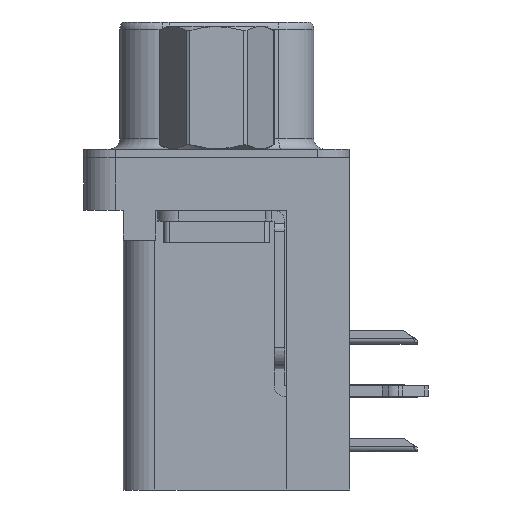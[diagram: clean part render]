
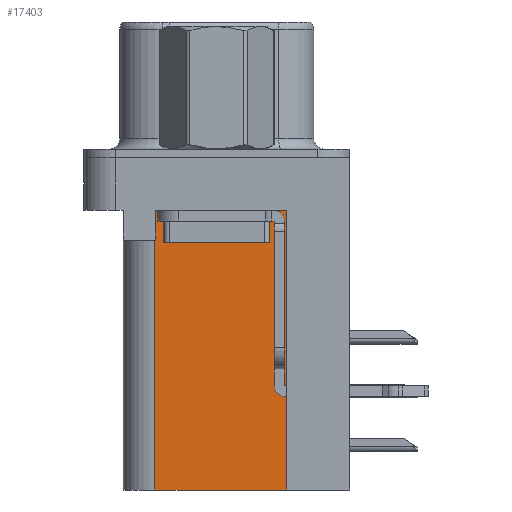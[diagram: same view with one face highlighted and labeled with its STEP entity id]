
A CAD part, left-side view. The second image highlights one B-rep face of the part: STEP entity #17403.
In plain terms, the highlighted planar face has unit normal (-1, 0, 0).
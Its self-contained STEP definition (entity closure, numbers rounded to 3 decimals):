
#1299 = ORIENTED_EDGE ( 'NONE', *, *, #2107, .T. ) ;
#1419 = ORIENTED_EDGE ( 'NONE', *, *, #11185, .T. ) ;
#1786 = LINE ( 'NONE', #12034, #20273 ) ;
#1880 = VECTOR ( 'NONE', #23965, 1000. ) ;
#2056 = EDGE_CURVE ( 'NONE', #6835, #28016, #26701, .T. ) ;
#2107 = EDGE_CURVE ( 'NONE', #3809, #8611, #20154, .T. ) ;
#2219 = CARTESIAN_POINT ( 'NONE',  ( 3.765, 2.925, -15.7 ) ) ;
#3132 = DIRECTION ( 'NONE',  ( 0., 0., -1. ) ) ;
#3398 = ORIENTED_EDGE ( 'NONE', *, *, #2056, .F. ) ;
#3809 = VERTEX_POINT ( 'NONE', #26616 ) ;
#4147 = CARTESIAN_POINT ( 'NONE',  ( 3.765, 2.925, -3.9 ) ) ;
#5010 = CARTESIAN_POINT ( 'NONE',  ( 3.765, 2.925, -15.7 ) ) ;
#6704 = LINE ( 'NONE', #8851, #17920 ) ;
#6835 = VERTEX_POINT ( 'NONE', #2219 ) ;
#7453 = CARTESIAN_POINT ( 'NONE',  ( 3.765, -3.295, -15.7 ) ) ;
#7613 = EDGE_CURVE ( 'NONE', #17355, #6835, #1786, .T. ) ;
#8280 = VECTOR ( 'NONE', #3132, 1000. ) ;
#8340 = CARTESIAN_POINT ( 'NONE',  ( 3.765, 2.895, -3.9 ) ) ;
#8611 = VERTEX_POINT ( 'NONE', #8340 ) ;
#8851 = CARTESIAN_POINT ( 'NONE',  ( 3.765, 0., -3.9 ) ) ;
#9215 = CARTESIAN_POINT ( 'NONE',  ( 3.765, -3.295, -2.5 ) ) ;
#10832 = EDGE_CURVE ( 'NONE', #17355, #16299, #27985, .T. ) ;
#11127 = DIRECTION ( 'NONE',  ( 0., 1., 0. ) ) ;
#11185 = EDGE_CURVE ( 'NONE', #16299, #3809, #20374, .T. ) ;
#12034 = CARTESIAN_POINT ( 'NONE',  ( 3.765, -3.295, -15.7 ) ) ;
#12742 = DIRECTION ( 'NONE',  ( 1., 0., 0. ) ) ;
#13169 = ORIENTED_EDGE ( 'NONE', *, *, #26629, .T. ) ;
#14181 = ORIENTED_EDGE ( 'NONE', *, *, #10832, .T. ) ;
#14394 = CARTESIAN_POINT ( 'NONE',  ( 3.765, 2.895, -3.9 ) ) ;
#14821 = CARTESIAN_POINT ( 'NONE',  ( 3.765, -3.295, -15.7 ) ) ;
#14981 = VECTOR ( 'NONE', #20861, 1000. ) ;
#16299 = VERTEX_POINT ( 'NONE', #9215 ) ;
#17355 = VERTEX_POINT ( 'NONE', #14821 ) ;
#17403 = ADVANCED_FACE ( 'NONE', ( #27098 ), #25972, .F. ) ;
#17920 = VECTOR ( 'NONE', #11127, 1000. ) ;
#20154 = LINE ( 'NONE', #14394, #8280 ) ;
#20273 = VECTOR ( 'NONE', #27531, 1000. ) ;
#20374 = LINE ( 'NONE', #21751, #1880 ) ;
#20629 = EDGE_LOOP ( 'NONE', ( #1419, #1299, #13169, #3398, #24075, #14181 ) ) ;
#20722 = VECTOR ( 'NONE', #25224, 1000. ) ;
#20861 = DIRECTION ( 'NONE',  ( 0., 0., 1. ) ) ;
#21751 = CARTESIAN_POINT ( 'NONE',  ( 3.765, -3.295, -2.5 ) ) ;
#23965 = DIRECTION ( 'NONE',  ( 0., 1., 0. ) ) ;
#24075 = ORIENTED_EDGE ( 'NONE', *, *, #7613, .F. ) ;
#25224 = DIRECTION ( 'NONE',  ( 0., 0., 1. ) ) ;
#25877 = CARTESIAN_POINT ( 'NONE',  ( 3.765, -3.295, -15.7 ) ) ;
#25972 = PLANE ( 'NONE',  #27710 ) ;
#26616 = CARTESIAN_POINT ( 'NONE',  ( 3.765, 2.895, -2.5 ) ) ;
#26629 = EDGE_CURVE ( 'NONE', #8611, #28016, #6704, .T. ) ;
#26701 = LINE ( 'NONE', #5010, #14981 ) ;
#27098 = FACE_OUTER_BOUND ( 'NONE', #20629, .T. ) ;
#27531 = DIRECTION ( 'NONE',  ( 0., 1., 0. ) ) ;
#27710 = AXIS2_PLACEMENT_3D ( 'NONE', #25877, #12742, #28225 ) ;
#27985 = LINE ( 'NONE', #7453, #20722 ) ;
#28016 = VERTEX_POINT ( 'NONE', #4147 ) ;
#28225 = DIRECTION ( 'NONE',  ( 0., 0., -1. ) ) ;
